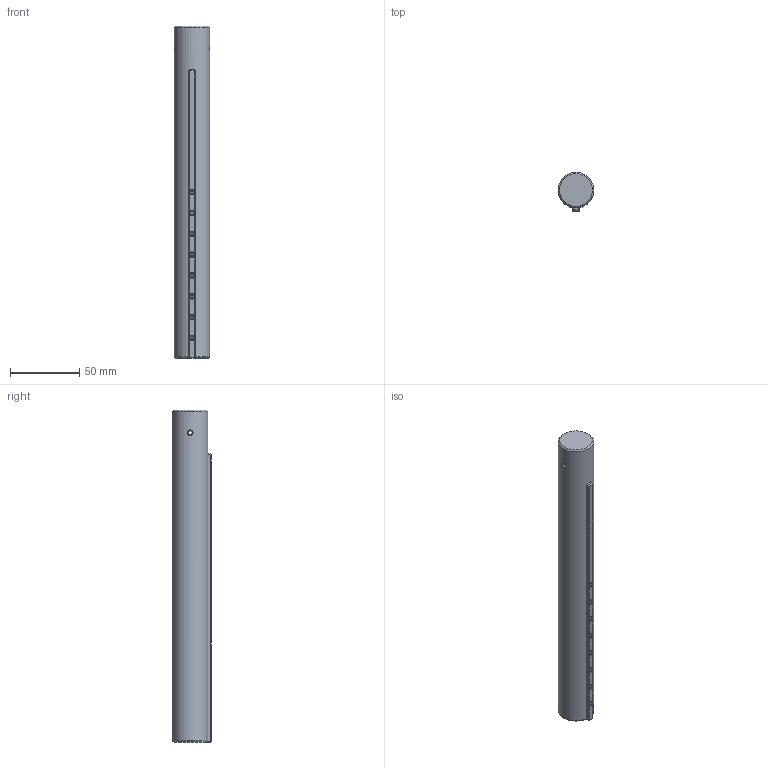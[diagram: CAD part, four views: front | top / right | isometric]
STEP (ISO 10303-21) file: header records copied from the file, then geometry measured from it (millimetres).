
FILE_DESCRIPTION(/* description */ (''),/* implementation_level */ '2;1');
FILE_NAME(/* name */ 'd8e3c478-4af0-4f16-8d6e-cf2f340f16ea.stp',/* time_stamp */ '2019-04-30T20:52:22-04:00',/* author */ ('suzuki450ltr'),/* organization */ (''),/* preprocessor_version */ 'ST-DEVELOPER v18',/* originating_system */ 'Autodesk Translation Framework v8.2.0.1029',/* authorisation */ '');
FILE_SCHEMA (('AUTOMOTIVE_DESIGN { 1 0 10303 214 3 1 1 }'));
Length unit declared in the file: millimetre
Products named in the file (1): Buffer Tube
Bounding box: 25.5 x 27.98 x 239.28 mm (x, y, z)
Volume: 124129.1 mm3; surface area: 21498.8 mm2
Topology: 1 solids, 1 shells, 64 faces, 164 edges, 101 vertices
Faces by surface type: plane 34, cone 17, cylinder 10, bspline 2, torus 1
Full cylindrical faces by diameter (mm): 3 x9, 25.5 x1
Entity records: 2281 total; most frequent: CARTESIAN_POINT 746, ORIENTED_EDGE 330, DIRECTION 303, EDGE_CURVE 165, AXIS2_PLACEMENT_3D 111, VERTEX_POINT 102, LINE 81, VECTOR 81
